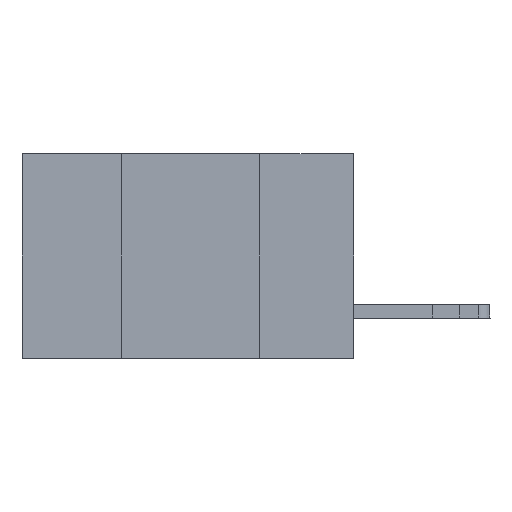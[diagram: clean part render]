
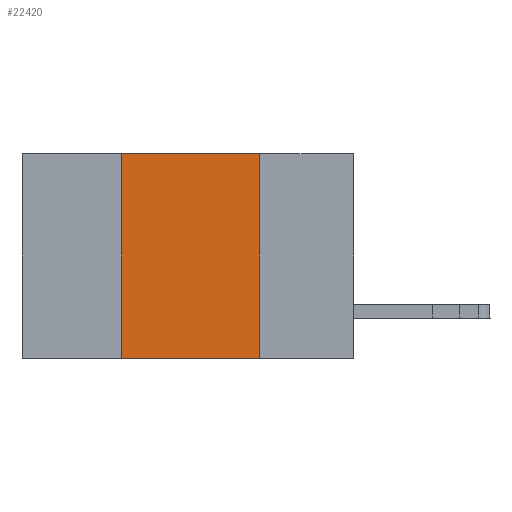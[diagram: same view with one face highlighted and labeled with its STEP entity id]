
A CAD part, left-side view. The second image highlights one B-rep face of the part: STEP entity #22420.
In plain terms, the highlighted planar face has unit normal (-1, 0, 0).
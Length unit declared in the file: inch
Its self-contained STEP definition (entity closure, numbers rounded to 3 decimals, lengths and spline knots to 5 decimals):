
#887 = LINE ( 'NONE', #12869, #21799 ) ;
#1206 = ORIENTED_EDGE ( 'NONE', *, *, #5785, .T. ) ;
#1403 = VERTEX_POINT ( 'NONE', #33869 ) ;
#4480 = PLANE ( 'NONE',  #30853 ) ;
#5785 = EDGE_CURVE ( 'NONE', #28319, #1403, #29961, .T. ) ;
#7314 = CARTESIAN_POINT ( 'NONE',  ( 0., 0.6, -0.37 ) ) ;
#7471 = VECTOR ( 'NONE', #17746, 39.37008 ) ;
#7591 = EDGE_CURVE ( 'NONE', #31495, #1403, #887, .T. ) ;
#11573 = VECTOR ( 'NONE', #26418, 39.37008 ) ;
#12544 = FACE_OUTER_BOUND ( 'NONE', #33026, .T. ) ;
#12780 = VECTOR ( 'NONE', #22329, 39.37008 ) ;
#12869 = CARTESIAN_POINT ( 'NONE',  ( 0., 0.17, 0. ) ) ;
#12993 = ORIENTED_EDGE ( 'NONE', *, *, #7591, .F. ) ;
#14074 = CARTESIAN_POINT ( 'NONE',  ( 0., 0.42, 0. ) ) ;
#15425 = CARTESIAN_POINT ( 'NONE',  ( 0., 0.6, 0. ) ) ;
#15518 = VERTEX_POINT ( 'NONE', #28840 ) ;
#17362 = EDGE_CURVE ( 'NONE', #15518, #31495, #29702, .T. ) ;
#17746 = DIRECTION ( 'NONE',  ( 0., -1., 0. ) ) ;
#18197 = DIRECTION ( 'NONE',  ( 1., 0., 0. ) ) ;
#18860 = EDGE_CURVE ( 'NONE', #28319, #15518, #20900, .T. ) ;
#19322 = CARTESIAN_POINT ( 'NONE',  ( 0., 0.6, 0. ) ) ;
#20900 = LINE ( 'NONE', #14074, #12780 ) ;
#21359 = DIRECTION ( 'NONE',  ( 0., 0., -1. ) ) ;
#21799 = VECTOR ( 'NONE', #21359, 39.37008 ) ;
#22329 = DIRECTION ( 'NONE',  ( 0., 0., 1. ) ) ;
#22420 = ADVANCED_FACE ( 'NONE', ( #12544 ), #4480, .F. ) ;
#23525 = ORIENTED_EDGE ( 'NONE', *, *, #17362, .F. ) ;
#25144 = CARTESIAN_POINT ( 'NONE',  ( 0., 0.17, 0. ) ) ;
#26418 = DIRECTION ( 'NONE',  ( 0., -1., 0. ) ) ;
#26531 = DIRECTION ( 'NONE',  ( 0., 0., -1. ) ) ;
#28319 = VERTEX_POINT ( 'NONE', #32169 ) ;
#28840 = CARTESIAN_POINT ( 'NONE',  ( 0., 0.42, 0. ) ) ;
#29702 = LINE ( 'NONE', #19322, #7471 ) ;
#29961 = LINE ( 'NONE', #7314, #11573 ) ;
#30853 = AXIS2_PLACEMENT_3D ( 'NONE', #15425, #18197, #26531 ) ;
#31495 = VERTEX_POINT ( 'NONE', #25144 ) ;
#32101 = ORIENTED_EDGE ( 'NONE', *, *, #18860, .F. ) ;
#32169 = CARTESIAN_POINT ( 'NONE',  ( 0., 0.42, -0.37 ) ) ;
#33026 = EDGE_LOOP ( 'NONE', ( #12993, #23525, #32101, #1206 ) ) ;
#33869 = CARTESIAN_POINT ( 'NONE',  ( 0., 0.17, -0.37 ) ) ;
